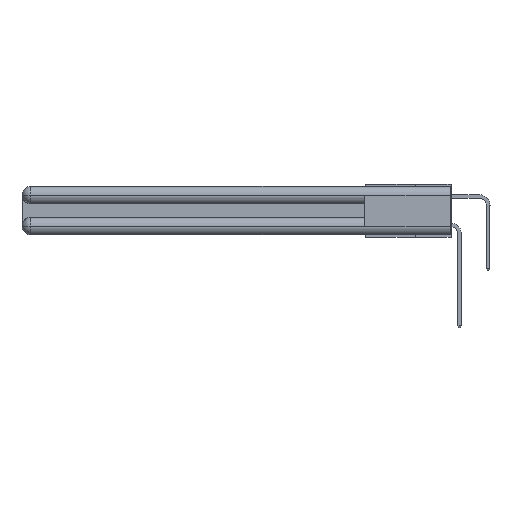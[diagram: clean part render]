
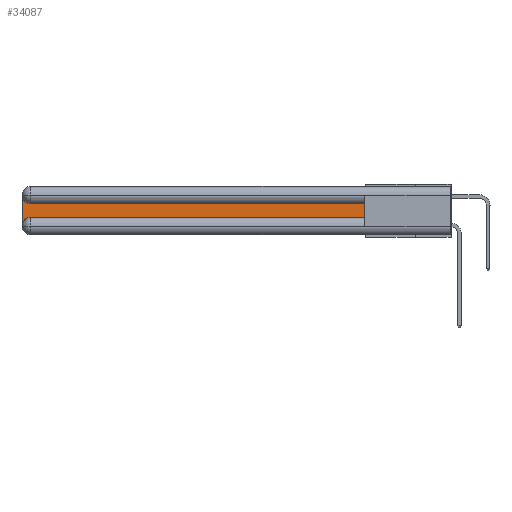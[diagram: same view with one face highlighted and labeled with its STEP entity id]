
A CAD part, left-side view. The second image highlights one B-rep face of the part: STEP entity #34087.
In plain terms, the highlighted planar face has unit normal (-1, 0, 0).
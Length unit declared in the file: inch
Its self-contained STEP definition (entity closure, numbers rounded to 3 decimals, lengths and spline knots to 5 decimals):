
#2306 = CARTESIAN_POINT ( 'NONE',  ( 0.075, 0.6, -0.2175 ) ) ;
#3121 = CARTESIAN_POINT ( 'NONE',  ( 0.075, 3., -0.2775 ) ) ;
#3263 = CIRCLE ( 'NONE', #32812, 0.06 ) ;
#3847 = ORIENTED_EDGE ( 'NONE', *, *, #31718, .T. ) ;
#4670 = LINE ( 'NONE', #33440, #34188 ) ;
#5567 = CIRCLE ( 'NONE', #32587, 0.06 ) ;
#5577 = LINE ( 'NONE', #31546, #24834 ) ;
#6225 = EDGE_CURVE ( 'NONE', #19718, #15022, #5577, .T. ) ;
#7901 = EDGE_LOOP ( 'NONE', ( #29701, #20411, #19747, #8589, #16238, #3847 ) ) ;
#8125 = VERTEX_POINT ( 'NONE', #36289 ) ;
#8589 = ORIENTED_EDGE ( 'NONE', *, *, #23170, .T. ) ;
#9498 = CARTESIAN_POINT ( 'NONE',  ( 0.075, 3., -0.2175 ) ) ;
#9758 = AXIS2_PLACEMENT_3D ( 'NONE', #24084, #16080, #16215 ) ;
#10248 = CARTESIAN_POINT ( 'NONE',  ( 0.075, 3., -0.0625 ) ) ;
#10509 = CARTESIAN_POINT ( 'NONE',  ( 0.075, 2.94, -0.1225 ) ) ;
#11085 = VERTEX_POINT ( 'NONE', #2306 ) ;
#11817 = VERTEX_POINT ( 'NONE', #10248 ) ;
#12022 = LINE ( 'NONE', #9498, #20541 ) ;
#15022 = VERTEX_POINT ( 'NONE', #10509 ) ;
#15803 = CARTESIAN_POINT ( 'NONE',  ( 0.075, 0.6, -0.2175 ) ) ;
#16080 = DIRECTION ( 'NONE',  ( 1., 0., 0. ) ) ;
#16215 = DIRECTION ( 'NONE',  ( 0., 0., -1. ) ) ;
#16238 = ORIENTED_EDGE ( 'NONE', *, *, #19632, .T. ) ;
#16328 = DIRECTION ( 'NONE',  ( 0., -1., 0. ) ) ;
#16584 = DIRECTION ( 'NONE',  ( 1., 0., 0. ) ) ;
#17334 = EDGE_CURVE ( 'NONE', #11817, #17690, #12022, .T. ) ;
#17690 = VERTEX_POINT ( 'NONE', #3121 ) ;
#18433 = CARTESIAN_POINT ( 'NONE',  ( 0.075, 2.94, -0.0625 ) ) ;
#19632 = EDGE_CURVE ( 'NONE', #8125, #11085, #4670, .T. ) ;
#19718 = VERTEX_POINT ( 'NONE', #22448 ) ;
#19747 = ORIENTED_EDGE ( 'NONE', *, *, #17334, .T. ) ;
#20274 = FACE_OUTER_BOUND ( 'NONE', #7901, .T. ) ;
#20411 = ORIENTED_EDGE ( 'NONE', *, *, #21688, .T. ) ;
#20541 = VECTOR ( 'NONE', #29273, 39.37008 ) ;
#21239 = PLANE ( 'NONE',  #9758 ) ;
#21688 = EDGE_CURVE ( 'NONE', #15022, #11817, #3263, .T. ) ;
#22448 = CARTESIAN_POINT ( 'NONE',  ( 0.075, 0.6, -0.1225 ) ) ;
#22586 = DIRECTION ( 'NONE',  ( 0., 0., -1. ) ) ;
#23073 = DIRECTION ( 'NONE',  ( 0., 1., 0. ) ) ;
#23170 = EDGE_CURVE ( 'NONE', #17690, #8125, #5567, .T. ) ;
#24041 = DIRECTION ( 'NONE',  ( 0., 0., -1. ) ) ;
#24084 = CARTESIAN_POINT ( 'NONE',  ( 0.075, 3., -0.1225 ) ) ;
#24834 = VECTOR ( 'NONE', #23073, 39.37008 ) ;
#24906 = DIRECTION ( 'NONE',  ( 0., 0., 1. ) ) ;
#28033 = LINE ( 'NONE', #15803, #32960 ) ;
#29273 = DIRECTION ( 'NONE',  ( 0., 0., -1. ) ) ;
#29701 = ORIENTED_EDGE ( 'NONE', *, *, #6225, .T. ) ;
#29769 = DIRECTION ( 'NONE',  ( 1., 0., 0. ) ) ;
#31546 = CARTESIAN_POINT ( 'NONE',  ( 0.075, 0.6, -0.1225 ) ) ;
#31718 = EDGE_CURVE ( 'NONE', #11085, #19718, #28033, .T. ) ;
#32587 = AXIS2_PLACEMENT_3D ( 'NONE', #36537, #16584, #22586 ) ;
#32812 = AXIS2_PLACEMENT_3D ( 'NONE', #18433, #29769, #24041 ) ;
#32960 = VECTOR ( 'NONE', #24906, 39.37008 ) ;
#33440 = CARTESIAN_POINT ( 'NONE',  ( 0.075, 0.6, -0.2175 ) ) ;
#34087 = ADVANCED_FACE ( 'NONE', ( #20274 ), #21239, .F. ) ;
#34188 = VECTOR ( 'NONE', #16328, 39.37008 ) ;
#36289 = CARTESIAN_POINT ( 'NONE',  ( 0.075, 2.94, -0.2175 ) ) ;
#36537 = CARTESIAN_POINT ( 'NONE',  ( 0.075, 2.94, -0.2775 ) ) ;
